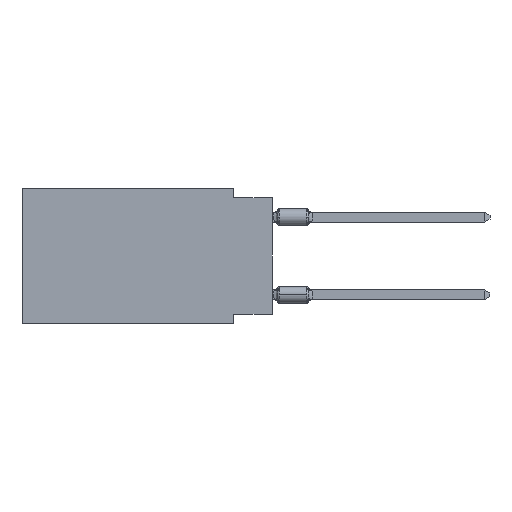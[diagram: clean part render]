
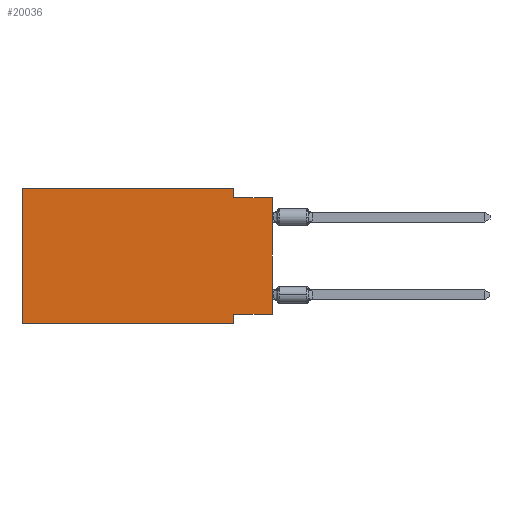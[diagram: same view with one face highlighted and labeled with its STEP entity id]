
A CAD part, left-side view. The second image highlights one B-rep face of the part: STEP entity #20036.
In plain terms, the highlighted planar face has unit normal (-1, 0, 0).
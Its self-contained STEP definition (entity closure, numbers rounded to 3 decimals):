
#298 = LINE ( 'NONE', #11739, #4644 ) ;
#458 = CARTESIAN_POINT ( 'NONE',  ( 0., 16.383, -8.89 ) ) ;
#1191 = CARTESIAN_POINT ( 'NONE',  ( 0., 0., -0.635 ) ) ;
#1346 = VERTEX_POINT ( 'NONE', #4568 ) ;
#1393 = EDGE_CURVE ( 'NONE', #12940, #18310, #6062, .T. ) ;
#1997 = EDGE_CURVE ( 'NONE', #12502, #2716, #14827, .T. ) ;
#2282 = VERTEX_POINT ( 'NONE', #2742 ) ;
#2331 = FACE_OUTER_BOUND ( 'NONE', #20856, .T. ) ;
#2548 = ORIENTED_EDGE ( 'NONE', *, *, #1997, .T. ) ;
#2716 = VERTEX_POINT ( 'NONE', #2826 ) ;
#2742 = CARTESIAN_POINT ( 'NONE',  ( 0., 2.54, -8.255 ) ) ;
#2826 = CARTESIAN_POINT ( 'NONE',  ( 0., 0., -0.635 ) ) ;
#3284 = CARTESIAN_POINT ( 'NONE',  ( 0., 0., -8.255 ) ) ;
#3758 = ORIENTED_EDGE ( 'NONE', *, *, #5288, .F. ) ;
#4568 = CARTESIAN_POINT ( 'NONE',  ( 0., 2.54, -8.89 ) ) ;
#4644 = VECTOR ( 'NONE', #10728, 1000. ) ;
#4937 = VECTOR ( 'NONE', #9011, 1000. ) ;
#4948 = CARTESIAN_POINT ( 'NONE',  ( 0., 2.54, -8.89 ) ) ;
#5159 = LINE ( 'NONE', #1191, #4937 ) ;
#5288 = EDGE_CURVE ( 'NONE', #12502, #2282, #12732, .T. ) ;
#5334 = CARTESIAN_POINT ( 'NONE',  ( 0., 16.383, 0. ) ) ;
#6062 = LINE ( 'NONE', #12289, #8587 ) ;
#6469 = AXIS2_PLACEMENT_3D ( 'NONE', #23295, #6897, #24146 ) ;
#6897 = DIRECTION ( 'NONE',  ( 1., 0., 0. ) ) ;
#7046 = ORIENTED_EDGE ( 'NONE', *, *, #14326, .F. ) ;
#7792 = LINE ( 'NONE', #458, #17862 ) ;
#8587 = VECTOR ( 'NONE', #17428, 1000. ) ;
#9011 = DIRECTION ( 'NONE',  ( 0., -1., 0. ) ) ;
#9021 = ORIENTED_EDGE ( 'NONE', *, *, #22229, .F. ) ;
#10312 = EDGE_CURVE ( 'NONE', #12378, #2716, #5159, .T. ) ;
#10557 = DIRECTION ( 'NONE',  ( 0., 0., -1. ) ) ;
#10728 = DIRECTION ( 'NONE',  ( 0., 0., -1. ) ) ;
#11714 = ORIENTED_EDGE ( 'NONE', *, *, #1393, .F. ) ;
#11739 = CARTESIAN_POINT ( 'NONE',  ( 0., 2.54, 0. ) ) ;
#11978 = CARTESIAN_POINT ( 'NONE',  ( 0., 16.383, 0. ) ) ;
#12289 = CARTESIAN_POINT ( 'NONE',  ( 0., 16.383, 0. ) ) ;
#12378 = VERTEX_POINT ( 'NONE', #18045 ) ;
#12502 = VERTEX_POINT ( 'NONE', #16655 ) ;
#12732 = LINE ( 'NONE', #3284, #14139 ) ;
#12940 = VERTEX_POINT ( 'NONE', #11978 ) ;
#13541 = ORIENTED_EDGE ( 'NONE', *, *, #16566, .T. ) ;
#14139 = VECTOR ( 'NONE', #22140, 1000. ) ;
#14326 = EDGE_CURVE ( 'NONE', #18310, #12378, #298, .T. ) ;
#14382 = VECTOR ( 'NONE', #14697, 1000. ) ;
#14697 = DIRECTION ( 'NONE',  ( 0., 0., 1. ) ) ;
#14709 = DIRECTION ( 'NONE',  ( 0., 0., 1. ) ) ;
#14827 = LINE ( 'NONE', #24239, #20593 ) ;
#16006 = VERTEX_POINT ( 'NONE', #16815 ) ;
#16300 = VECTOR ( 'NONE', #10557, 1000. ) ;
#16566 = EDGE_CURVE ( 'NONE', #16006, #1346, #7792, .T. ) ;
#16655 = CARTESIAN_POINT ( 'NONE',  ( 0., 0., -8.255 ) ) ;
#16815 = CARTESIAN_POINT ( 'NONE',  ( 0., 16.383, -8.89 ) ) ;
#17428 = DIRECTION ( 'NONE',  ( 0., -1., 0. ) ) ;
#17529 = PLANE ( 'NONE',  #6469 ) ;
#17574 = EDGE_CURVE ( 'NONE', #2282, #1346, #23829, .T. ) ;
#17862 = VECTOR ( 'NONE', #23065, 1000. ) ;
#18045 = CARTESIAN_POINT ( 'NONE',  ( 0., 2.54, -0.635 ) ) ;
#18310 = VERTEX_POINT ( 'NONE', #19886 ) ;
#19886 = CARTESIAN_POINT ( 'NONE',  ( 0., 2.54, 0. ) ) ;
#20036 = ADVANCED_FACE ( 'NONE', ( #2331 ), #17529, .F. ) ;
#20593 = VECTOR ( 'NONE', #14709, 1000. ) ;
#20822 = LINE ( 'NONE', #5334, #14382 ) ;
#20856 = EDGE_LOOP ( 'NONE', ( #2548, #21854, #7046, #11714, #9021, #13541, #22291, #3758 ) ) ;
#21854 = ORIENTED_EDGE ( 'NONE', *, *, #10312, .F. ) ;
#22140 = DIRECTION ( 'NONE',  ( 0., 1., 0. ) ) ;
#22229 = EDGE_CURVE ( 'NONE', #16006, #12940, #20822, .T. ) ;
#22291 = ORIENTED_EDGE ( 'NONE', *, *, #17574, .F. ) ;
#23065 = DIRECTION ( 'NONE',  ( 0., -1., 0. ) ) ;
#23295 = CARTESIAN_POINT ( 'NONE',  ( 0., 16.383, 0. ) ) ;
#23829 = LINE ( 'NONE', #4948, #16300 ) ;
#24146 = DIRECTION ( 'NONE',  ( 0., 0., -1. ) ) ;
#24239 = CARTESIAN_POINT ( 'NONE',  ( 0., 0., 0. ) ) ;
